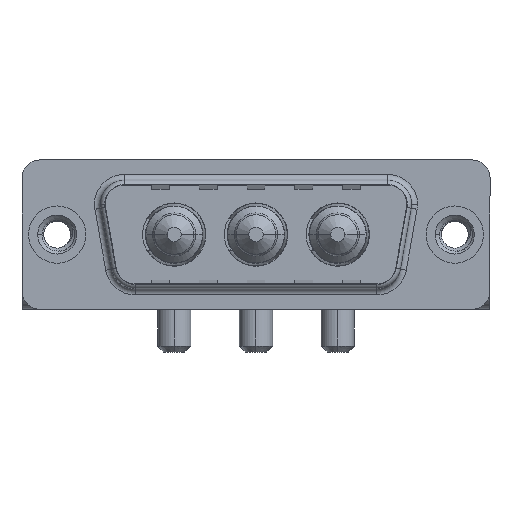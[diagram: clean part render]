
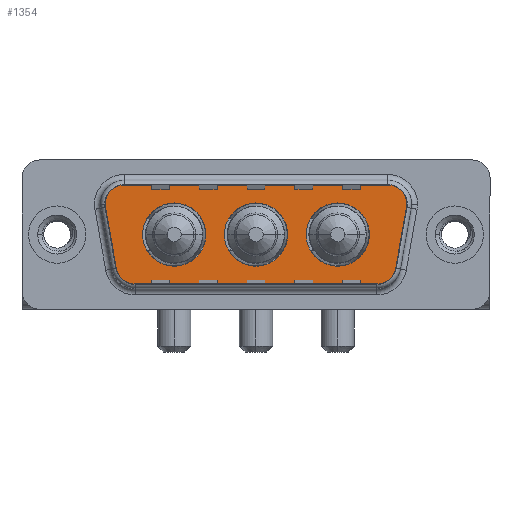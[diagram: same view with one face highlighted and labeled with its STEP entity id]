
A CAD part, top view. The second image highlights one B-rep face of the part: STEP entity #1354.
In plain terms, the highlighted planar face has unit normal (0, 0, 1).
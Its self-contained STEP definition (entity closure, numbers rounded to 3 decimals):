
#30 = FACE_BOUND ( 'NONE', #5540, .T. ) ;
#63 = LINE ( 'NONE', #12836, #5253 ) ;
#227 = CIRCLE ( 'NONE', #7918, 2. ) ;
#322 = VERTEX_POINT ( 'NONE', #12566 ) ;
#560 = EDGE_CURVE ( 'NONE', #8153, #9775, #63, .T. ) ;
#653 = VERTEX_POINT ( 'NONE', #13240 ) ;
#821 = CARTESIAN_POINT ( 'NONE',  ( 4.464, -3.247, 0. ) ) ;
#866 = LINE ( 'NONE', #12412, #3740 ) ;
#912 = AXIS2_PLACEMENT_3D ( 'NONE', #1216, #8334, #4193 ) ;
#1102 = EDGE_CURVE ( 'NONE', #9775, #3068, #3070, .T. ) ;
#1216 = CARTESIAN_POINT ( 'NONE',  ( 16.65, 0., 0. ) ) ;
#1307 = EDGE_CURVE ( 'NONE', #653, #1359, #5934, .T. ) ;
#1335 = CARTESIAN_POINT ( 'NONE',  ( 6.434, -4.9, 0. ) ) ;
#1340 = CIRCLE ( 'NONE', #9059, 2. ) ;
#1354 = ADVANCED_FACE ( 'NONE', ( #5310, #30, #10450, #12799 ), #4223, .T. ) ;
#1359 = VERTEX_POINT ( 'NONE', #9690 ) ;
#1375 = VERTEX_POINT ( 'NONE', #12669 ) ;
#1474 = CARTESIAN_POINT ( 'NONE',  ( 6.434, -2.9, 0. ) ) ;
#2180 = ORIENTED_EDGE ( 'NONE', *, *, #7374, .T. ) ;
#2208 = DIRECTION ( 'NONE',  ( 0., 0., 1. ) ) ;
#2266 = DIRECTION ( 'NONE',  ( 1., 0., 0. ) ) ;
#2336 = CARTESIAN_POINT ( 'NONE',  ( 9.8, 0., 0. ) ) ;
#2430 = CARTESIAN_POINT ( 'NONE',  ( 5.411, 2.9, 0. ) ) ;
#2632 = DIRECTION ( 'NONE',  ( 0., 0., 1. ) ) ;
#2663 = VERTEX_POINT ( 'NONE', #6009 ) ;
#2672 = ORIENTED_EDGE ( 'NONE', *, *, #9580, .T. ) ;
#2929 = CIRCLE ( 'NONE', #13530, 2.65 ) ;
#3067 = EDGE_CURVE ( 'NONE', #9958, #11633, #9763, .T. ) ;
#3068 = VERTEX_POINT ( 'NONE', #1335 ) ;
#3070 = CIRCLE ( 'NONE', #3734, 2. ) ;
#3124 = CARTESIAN_POINT ( 'NONE',  ( 29.859, 2.553, 0. ) ) ;
#3353 = ORIENTED_EDGE ( 'NONE', *, *, #9783, .T. ) ;
#3383 = DIRECTION ( 'NONE',  ( 1., 0., 0. ) ) ;
#3425 = DIRECTION ( 'NONE',  ( 0.174, -0.985, 0. ) ) ;
#3501 = EDGE_CURVE ( 'NONE', #5948, #12074, #2929, .T. ) ;
#3727 = CARTESIAN_POINT ( 'NONE',  ( 5.411, 4.9, 0. ) ) ;
#3734 = AXIS2_PLACEMENT_3D ( 'NONE', #1474, #2632, #7677 ) ;
#3740 = VECTOR ( 'NONE', #7204, 1000. ) ;
#3925 = CARTESIAN_POINT ( 'NONE',  ( 27.889, 4.9, 0. ) ) ;
#3943 = DIRECTION ( 'NONE',  ( 0., 0., 1. ) ) ;
#4112 = ORIENTED_EDGE ( 'NONE', *, *, #7066, .F. ) ;
#4149 = DIRECTION ( 'NONE',  ( 0., 0., 1. ) ) ;
#4193 = DIRECTION ( 'NONE',  ( 1., 0., 0. ) ) ;
#4206 = CIRCLE ( 'NONE', #912, 2.65 ) ;
#4223 = PLANE ( 'NONE',  #7502 ) ;
#4605 = DIRECTION ( 'NONE',  ( 0., 0., 1. ) ) ;
#5042 = AXIS2_PLACEMENT_3D ( 'NONE', #2336, #11595, #2266 ) ;
#5228 = EDGE_CURVE ( 'NONE', #1375, #2663, #227, .T. ) ;
#5253 = VECTOR ( 'NONE', #3425, 1000. ) ;
#5310 = FACE_BOUND ( 'NONE', #6354, .T. ) ;
#5383 = DIRECTION ( 'NONE',  ( 0.174, 0.985, 0. ) ) ;
#5496 = CARTESIAN_POINT ( 'NONE',  ( 3.441, 2.553, 0. ) ) ;
#5540 = EDGE_LOOP ( 'NONE', ( #8467, #7551 ) ) ;
#5718 = DIRECTION ( 'NONE',  ( 0., 0., 1. ) ) ;
#5920 = CIRCLE ( 'NONE', #5042, 2.65 ) ;
#5934 = CIRCLE ( 'NONE', #9053, 2.65 ) ;
#5948 = VERTEX_POINT ( 'NONE', #12522 ) ;
#6009 = CARTESIAN_POINT ( 'NONE',  ( 29.889, 2.9, 0. ) ) ;
#6109 = EDGE_CURVE ( 'NONE', #7824, #8153, #11135, .T. ) ;
#6219 = DIRECTION ( 'NONE',  ( 1., 0., 0. ) ) ;
#6225 = CARTESIAN_POINT ( 'NONE',  ( 23.5, 0., 0. ) ) ;
#6354 = EDGE_LOOP ( 'NONE', ( #11009, #11582 ) ) ;
#6397 = DIRECTION ( 'NONE',  ( -1., 0., 0. ) ) ;
#6424 = LINE ( 'NONE', #3124, #12820 ) ;
#6628 = CARTESIAN_POINT ( 'NONE',  ( 12.45, 0., 0. ) ) ;
#6693 = DIRECTION ( 'NONE',  ( 1., 0., 0. ) ) ;
#6984 = EDGE_CURVE ( 'NONE', #3068, #322, #9730, .T. ) ;
#7036 = AXIS2_PLACEMENT_3D ( 'NONE', #11607, #11742, #8632 ) ;
#7066 = EDGE_CURVE ( 'NONE', #12074, #5948, #5920, .T. ) ;
#7204 = DIRECTION ( 'NONE',  ( -1., 0., 0. ) ) ;
#7251 = VECTOR ( 'NONE', #12705, 1000. ) ;
#7339 = ORIENTED_EDGE ( 'NONE', *, *, #560, .T. ) ;
#7374 = EDGE_CURVE ( 'NONE', #12263, #7824, #866, .T. ) ;
#7456 = DIRECTION ( 'NONE',  ( 0., 0., 1. ) ) ;
#7496 = CIRCLE ( 'NONE', #7036, 2. ) ;
#7502 = AXIS2_PLACEMENT_3D ( 'NONE', #8440, #7456, #10515 ) ;
#7551 = ORIENTED_EDGE ( 'NONE', *, *, #1307, .F. ) ;
#7577 = CARTESIAN_POINT ( 'NONE',  ( 6.434, -4.9, 0. ) ) ;
#7627 = EDGE_CURVE ( 'NONE', #2663, #12263, #7496, .T. ) ;
#7677 = DIRECTION ( 'NONE',  ( -1., 0., 0. ) ) ;
#7681 = CARTESIAN_POINT ( 'NONE',  ( 28.836, -3.247, 0. ) ) ;
#7824 = VERTEX_POINT ( 'NONE', #3727 ) ;
#7840 = ORIENTED_EDGE ( 'NONE', *, *, #1102, .T. ) ;
#7911 = ORIENTED_EDGE ( 'NONE', *, *, #6109, .T. ) ;
#7918 = AXIS2_PLACEMENT_3D ( 'NONE', #11668, #2208, #6397 ) ;
#7943 = DIRECTION ( 'NONE',  ( 1., 0., 0. ) ) ;
#7959 = AXIS2_PLACEMENT_3D ( 'NONE', #6225, #3943, #12396 ) ;
#8153 = VERTEX_POINT ( 'NONE', #5496 ) ;
#8334 = DIRECTION ( 'NONE',  ( 0., 0., 1. ) ) ;
#8440 = CARTESIAN_POINT ( 'NONE',  ( 26.866, -2.9, 0. ) ) ;
#8467 = ORIENTED_EDGE ( 'NONE', *, *, #10664, .F. ) ;
#8632 = DIRECTION ( 'NONE',  ( -1., 0., 0. ) ) ;
#8921 = CARTESIAN_POINT ( 'NONE',  ( 16.65, 0., 0. ) ) ;
#8949 = EDGE_LOOP ( 'NONE', ( #3353, #2672, #9441, #10865, #2180, #7911, #7339, #7840, #12849 ) ) ;
#9053 = AXIS2_PLACEMENT_3D ( 'NONE', #11688, #4149, #6219 ) ;
#9059 = AXIS2_PLACEMENT_3D ( 'NONE', #12637, #13601, #11316 ) ;
#9441 = ORIENTED_EDGE ( 'NONE', *, *, #5228, .T. ) ;
#9580 = EDGE_CURVE ( 'NONE', #10414, #1375, #6424, .T. ) ;
#9690 = CARTESIAN_POINT ( 'NONE',  ( 26.15, 0., 0. ) ) ;
#9730 = LINE ( 'NONE', #7577, #7251 ) ;
#9763 = CIRCLE ( 'NONE', #11085, 2.65 ) ;
#9775 = VERTEX_POINT ( 'NONE', #821 ) ;
#9783 = EDGE_CURVE ( 'NONE', #322, #10414, #1340, .T. ) ;
#9830 = DIRECTION ( 'NONE',  ( 0., 0., 1. ) ) ;
#9841 = EDGE_CURVE ( 'NONE', #11633, #9958, #4206, .T. ) ;
#9958 = VERTEX_POINT ( 'NONE', #11659 ) ;
#10414 = VERTEX_POINT ( 'NONE', #7681 ) ;
#10450 = FACE_BOUND ( 'NONE', #11739, .T. ) ;
#10471 = AXIS2_PLACEMENT_3D ( 'NONE', #2430, #9830, #6693 ) ;
#10515 = DIRECTION ( 'NONE',  ( 1., 0., 0. ) ) ;
#10664 = EDGE_CURVE ( 'NONE', #1359, #653, #12168, .T. ) ;
#10865 = ORIENTED_EDGE ( 'NONE', *, *, #7627, .T. ) ;
#10979 = CARTESIAN_POINT ( 'NONE',  ( 9.8, 0., 0. ) ) ;
#11009 = ORIENTED_EDGE ( 'NONE', *, *, #3067, .F. ) ;
#11041 = ORIENTED_EDGE ( 'NONE', *, *, #3501, .F. ) ;
#11085 = AXIS2_PLACEMENT_3D ( 'NONE', #8921, #5718, #7943 ) ;
#11135 = CIRCLE ( 'NONE', #10471, 2. ) ;
#11148 = CARTESIAN_POINT ( 'NONE',  ( 14., 0., 0. ) ) ;
#11316 = DIRECTION ( 'NONE',  ( 1., 0., 0. ) ) ;
#11582 = ORIENTED_EDGE ( 'NONE', *, *, #9841, .F. ) ;
#11595 = DIRECTION ( 'NONE',  ( 0., 0., 1. ) ) ;
#11607 = CARTESIAN_POINT ( 'NONE',  ( 27.889, 2.9, 0. ) ) ;
#11633 = VERTEX_POINT ( 'NONE', #11148 ) ;
#11659 = CARTESIAN_POINT ( 'NONE',  ( 19.3, 0., 0. ) ) ;
#11668 = CARTESIAN_POINT ( 'NONE',  ( 27.889, 2.9, 0. ) ) ;
#11688 = CARTESIAN_POINT ( 'NONE',  ( 23.5, 0., 0. ) ) ;
#11739 = EDGE_LOOP ( 'NONE', ( #4112, #11041 ) ) ;
#11742 = DIRECTION ( 'NONE',  ( 0., 0., 1. ) ) ;
#12074 = VERTEX_POINT ( 'NONE', #6628 ) ;
#12168 = CIRCLE ( 'NONE', #7959, 2.65 ) ;
#12263 = VERTEX_POINT ( 'NONE', #3925 ) ;
#12396 = DIRECTION ( 'NONE',  ( 1., 0., 0. ) ) ;
#12412 = CARTESIAN_POINT ( 'NONE',  ( 5.411, 4.9, 0. ) ) ;
#12522 = CARTESIAN_POINT ( 'NONE',  ( 7.15, 0., 0. ) ) ;
#12566 = CARTESIAN_POINT ( 'NONE',  ( 26.866, -4.9, 0. ) ) ;
#12637 = CARTESIAN_POINT ( 'NONE',  ( 26.866, -2.9, 0. ) ) ;
#12669 = CARTESIAN_POINT ( 'NONE',  ( 29.859, 2.553, 0. ) ) ;
#12705 = DIRECTION ( 'NONE',  ( 1., 0., 0. ) ) ;
#12799 = FACE_OUTER_BOUND ( 'NONE', #8949, .T. ) ;
#12820 = VECTOR ( 'NONE', #5383, 1000. ) ;
#12836 = CARTESIAN_POINT ( 'NONE',  ( 3.441, 2.553, 0. ) ) ;
#12849 = ORIENTED_EDGE ( 'NONE', *, *, #6984, .T. ) ;
#13240 = CARTESIAN_POINT ( 'NONE',  ( 20.85, 0., 0. ) ) ;
#13530 = AXIS2_PLACEMENT_3D ( 'NONE', #10979, #4605, #3383 ) ;
#13601 = DIRECTION ( 'NONE',  ( 0., 0., 1. ) ) ;
